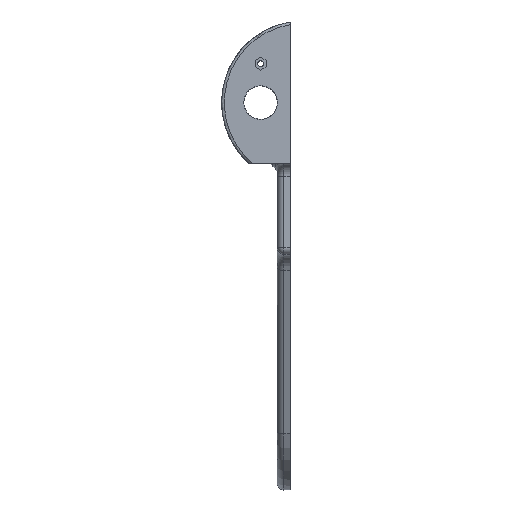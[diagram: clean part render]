
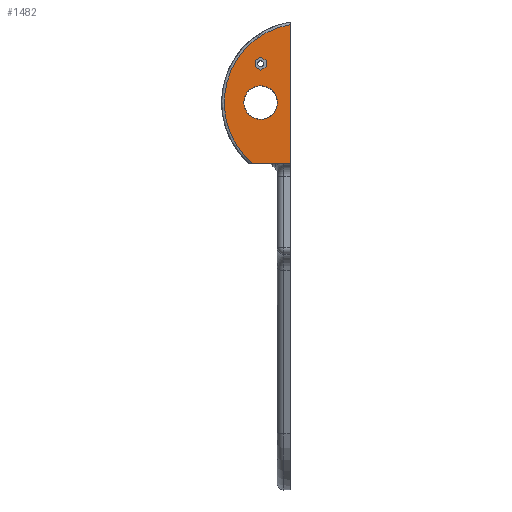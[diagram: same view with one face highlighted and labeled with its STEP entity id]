
A CAD part, top view. The second image highlights one B-rep face of the part: STEP entity #1482.
In plain terms, the highlighted planar face has unit normal (0, 0, 1).
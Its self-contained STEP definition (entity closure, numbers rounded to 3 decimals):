
#19 = FACE_OUTER_BOUND ( 'NONE', #1327, .T. ) ;
#38 = VERTEX_POINT ( 'NONE', #3658 ) ;
#92 = DIRECTION ( 'NONE',  ( 0., 1., 0. ) ) ;
#113 = CARTESIAN_POINT ( 'NONE',  ( 10., 3.534, 35. ) ) ;
#271 = CARTESIAN_POINT ( 'NONE',  ( -6.466, 3.534, 35. ) ) ;
#325 = ORIENTED_EDGE ( 'NONE', *, *, #500, .F. ) ;
#459 = ORIENTED_EDGE ( 'NONE', *, *, #2997, .F. ) ;
#483 = VECTOR ( 'NONE', #1606, 1000. ) ;
#500 = EDGE_CURVE ( 'NONE', #2054, #2285, #2684, .T. ) ;
#543 = DIRECTION ( 'NONE',  ( 0., 1., 0. ) ) ;
#693 = DIRECTION ( 'NONE',  ( 1., 0., 0. ) ) ;
#722 = LINE ( 'NONE', #4268, #856 ) ;
#738 = DIRECTION ( 'NONE',  ( -0.866, 0.5, 0. ) ) ;
#774 = ORIENTED_EDGE ( 'NONE', *, *, #2844, .F. ) ;
#856 = VECTOR ( 'NONE', #1887, 1000. ) ;
#918 = LINE ( 'NONE', #3313, #1862 ) ;
#980 = DIRECTION ( 'NONE',  ( -1., 0., 0. ) ) ;
#1058 = LINE ( 'NONE', #4450, #5094 ) ;
#1135 = FACE_BOUND ( 'NONE', #3267, .T. ) ;
#1220 = CARTESIAN_POINT ( 'NONE',  ( -8.591, 17.307, 35. ) ) ;
#1231 = ORIENTED_EDGE ( 'NONE', *, *, #2062, .F. ) ;
#1289 = VERTEX_POINT ( 'NONE', #5096 ) ;
#1308 = AXIS2_PLACEMENT_3D ( 'NONE', #4498, #2516, #92 ) ;
#1326 = PLANE ( 'NONE',  #1308 ) ;
#1327 = EDGE_LOOP ( 'NONE', ( #2070, #774, #3068 ) ) ;
#1347 = DIRECTION ( 'NONE',  ( 0.866, 0.5, 0. ) ) ;
#1366 = VERTEX_POINT ( 'NONE', #1645 ) ;
#1454 = VERTEX_POINT ( 'NONE', #3693 ) ;
#1459 = CARTESIAN_POINT ( 'NONE',  ( -4.341, 19.76, 35. ) ) ;
#1482 = ADVANCED_FACE ( 'NONE', ( #1135, #2080, #19 ), #1326, .F. ) ;
#1564 = LINE ( 'NONE', #4753, #483 ) ;
#1596 = DIRECTION ( 'NONE',  ( 0., -1., 0. ) ) ;
#1606 = DIRECTION ( 'NONE',  ( 0., -1., 0. ) ) ;
#1645 = CARTESIAN_POINT ( 'NONE',  ( -8.591, 19.76, 35. ) ) ;
#1741 = CIRCLE ( 'NONE', #3308, 30.5 ) ;
#1796 = EDGE_CURVE ( 'NONE', #1289, #1946, #4255, .T. ) ;
#1862 = VECTOR ( 'NONE', #1347, 1000. ) ;
#1869 = VERTEX_POINT ( 'NONE', #1459 ) ;
#1887 = DIRECTION ( 'NONE',  ( 0., 1., 0. ) ) ;
#1946 = VERTEX_POINT ( 'NONE', #3925 ) ;
#1965 = ORIENTED_EDGE ( 'NONE', *, *, #2208, .F. ) ;
#2054 = VERTEX_POINT ( 'NONE', #3579 ) ;
#2062 = EDGE_CURVE ( 'NONE', #1366, #1289, #1564, .T. ) ;
#2070 = ORIENTED_EDGE ( 'NONE', *, *, #2314, .T. ) ;
#2080 = FACE_BOUND ( 'NONE', #2434, .T. ) ;
#2128 = CARTESIAN_POINT ( 'NONE',  ( -12.933, 3.534, 35. ) ) ;
#2172 = CARTESIAN_POINT ( 'NONE',  ( 5., -20., 35. ) ) ;
#2207 = CARTESIAN_POINT ( 'NONE',  ( -6.466, 3.534, 35. ) ) ;
#2208 = EDGE_CURVE ( 'NONE', #1454, #1366, #1058, .T. ) ;
#2285 = VERTEX_POINT ( 'NONE', #2128 ) ;
#2314 = EDGE_CURVE ( 'NONE', #38, #4298, #1741, .T. ) ;
#2367 = VERTEX_POINT ( 'NONE', #2953 ) ;
#2434 = EDGE_LOOP ( 'NONE', ( #325, #3892 ) ) ;
#2460 = EDGE_CURVE ( 'NONE', #1869, #1454, #4519, .T. ) ;
#2516 = DIRECTION ( 'NONE',  ( 0., 0., -1. ) ) ;
#2583 = CIRCLE ( 'NONE', #5075, 6.466 ) ;
#2599 = DIRECTION ( 'NONE',  ( 1., 0., 0. ) ) ;
#2654 = CARTESIAN_POINT ( 'NONE',  ( 5., -20., 35. ) ) ;
#2684 = CIRCLE ( 'NONE', #3092, 6.466 ) ;
#2844 = EDGE_CURVE ( 'NONE', #3966, #4298, #4400, .T. ) ;
#2861 = DIRECTION ( 'NONE',  ( -0.866, -0.5, 0. ) ) ;
#2936 = DIRECTION ( 'NONE',  ( 0., 0., 1. ) ) ;
#2953 = CARTESIAN_POINT ( 'NONE',  ( -4.341, 17.307, 35. ) ) ;
#2997 = EDGE_CURVE ( 'NONE', #2367, #1869, #722, .T. ) ;
#3066 = VECTOR ( 'NONE', #1596, 1000. ) ;
#3068 = ORIENTED_EDGE ( 'NONE', *, *, #4756, .F. ) ;
#3071 = DIRECTION ( 'NONE',  ( 0., 0., 1. ) ) ;
#3092 = AXIS2_PLACEMENT_3D ( 'NONE', #271, #3071, #693 ) ;
#3161 = CARTESIAN_POINT ( 'NONE',  ( 5., 0., 35. ) ) ;
#3257 = EDGE_CURVE ( 'NONE', #1946, #2367, #918, .T. ) ;
#3267 = EDGE_LOOP ( 'NONE', ( #1965, #3918, #459, #4913, #4762, #1231 ) ) ;
#3308 = AXIS2_PLACEMENT_3D ( 'NONE', #113, #2936, #543 ) ;
#3313 = CARTESIAN_POINT ( 'NONE',  ( -6.466, 16.08, 35. ) ) ;
#3579 = CARTESIAN_POINT ( 'NONE',  ( 0., 3.534, 35. ) ) ;
#3658 = CARTESIAN_POINT ( 'NONE',  ( 5., 33.621, 35. ) ) ;
#3693 = CARTESIAN_POINT ( 'NONE',  ( -6.466, 20.987, 35. ) ) ;
#3726 = EDGE_CURVE ( 'NONE', #2285, #2054, #2583, .T. ) ;
#3892 = ORIENTED_EDGE ( 'NONE', *, *, #3726, .F. ) ;
#3918 = ORIENTED_EDGE ( 'NONE', *, *, #2460, .F. ) ;
#3925 = CARTESIAN_POINT ( 'NONE',  ( -6.466, 16.08, 35. ) ) ;
#3966 = VERTEX_POINT ( 'NONE', #2654 ) ;
#4003 = CARTESIAN_POINT ( 'NONE',  ( -9.402, -20., 35. ) ) ;
#4130 = VECTOR ( 'NONE', #4399, 1000. ) ;
#4146 = LINE ( 'NONE', #3161, #3066 ) ;
#4255 = LINE ( 'NONE', #1220, #4130 ) ;
#4268 = CARTESIAN_POINT ( 'NONE',  ( -4.341, 17.307, 35. ) ) ;
#4289 = VECTOR ( 'NONE', #738, 1000. ) ;
#4298 = VERTEX_POINT ( 'NONE', #4003 ) ;
#4314 = CARTESIAN_POINT ( 'NONE',  ( -4.341, 19.76, 35. ) ) ;
#4399 = DIRECTION ( 'NONE',  ( 0.866, -0.5, 0. ) ) ;
#4400 = LINE ( 'NONE', #2172, #5140 ) ;
#4450 = CARTESIAN_POINT ( 'NONE',  ( -6.466, 20.987, 35. ) ) ;
#4498 = CARTESIAN_POINT ( 'NONE',  ( 5., 0., 35. ) ) ;
#4519 = LINE ( 'NONE', #4314, #4289 ) ;
#4753 = CARTESIAN_POINT ( 'NONE',  ( -8.591, 19.76, 35. ) ) ;
#4756 = EDGE_CURVE ( 'NONE', #38, #3966, #4146, .T. ) ;
#4762 = ORIENTED_EDGE ( 'NONE', *, *, #1796, .F. ) ;
#4913 = ORIENTED_EDGE ( 'NONE', *, *, #3257, .F. ) ;
#4962 = DIRECTION ( 'NONE',  ( 0., 0., 1. ) ) ;
#5075 = AXIS2_PLACEMENT_3D ( 'NONE', #2207, #4962, #2599 ) ;
#5094 = VECTOR ( 'NONE', #2861, 1000. ) ;
#5096 = CARTESIAN_POINT ( 'NONE',  ( -8.591, 17.307, 35. ) ) ;
#5140 = VECTOR ( 'NONE', #980, 1000. ) ;
